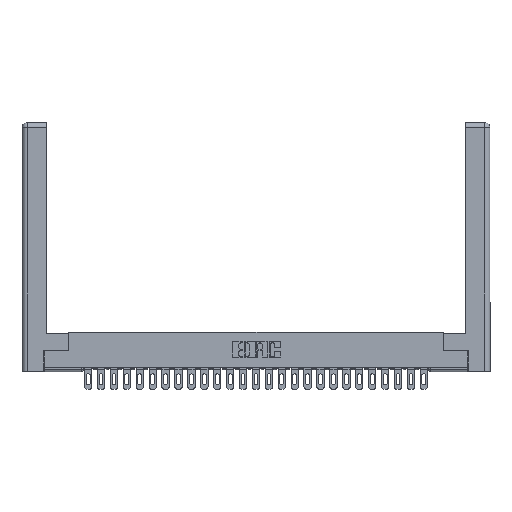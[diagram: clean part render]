
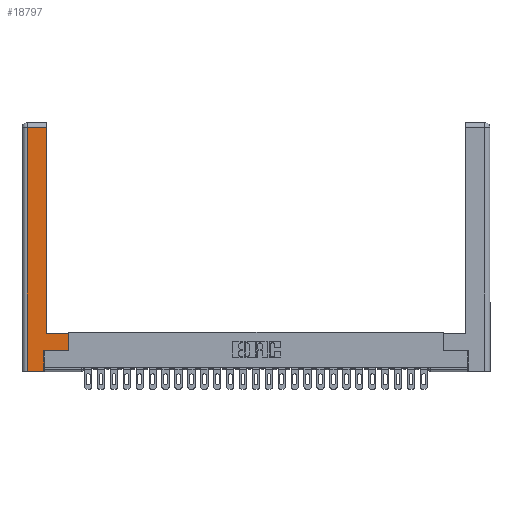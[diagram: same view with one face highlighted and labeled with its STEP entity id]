
A CAD part, top view. The second image highlights one B-rep face of the part: STEP entity #18797.
In plain terms, the highlighted planar face has unit normal (0, 0, 1).
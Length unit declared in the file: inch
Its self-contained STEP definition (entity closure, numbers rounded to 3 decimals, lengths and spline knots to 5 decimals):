
#316 = ORIENTED_EDGE ( 'NONE', *, *, #25225, .T. ) ;
#901 = VECTOR ( 'NONE', #3980, 39.37008 ) ;
#1416 = VERTEX_POINT ( 'NONE', #12453 ) ;
#1665 = VECTOR ( 'NONE', #17833, 39.37008 ) ;
#2496 = VECTOR ( 'NONE', #4115, 39.37008 ) ;
#3275 = VERTEX_POINT ( 'NONE', #26505 ) ;
#3876 = VECTOR ( 'NONE', #23729, 39.37008 ) ;
#3980 = DIRECTION ( 'NONE',  ( 1., 0., 0. ) ) ;
#4115 = DIRECTION ( 'NONE',  ( 0., 1., 0. ) ) ;
#4447 = CARTESIAN_POINT ( 'NONE',  ( 0., 0., 0. ) ) ;
#4611 = ORIENTED_EDGE ( 'NONE', *, *, #17147, .T. ) ;
#5420 = ORIENTED_EDGE ( 'NONE', *, *, #26320, .T. ) ;
#5506 = DIRECTION ( 'NONE',  ( -1., 0., 0. ) ) ;
#5956 = LINE ( 'NONE', #10548, #8752 ) ;
#5998 = LINE ( 'NONE', #8160, #2496 ) ;
#6754 = CARTESIAN_POINT ( 'NONE',  ( 0.565, 0.245, 0. ) ) ;
#7474 = EDGE_CURVE ( 'NONE', #3275, #1416, #10131, .T. ) ;
#7957 = LINE ( 'NONE', #8093, #10818 ) ;
#8093 = CARTESIAN_POINT ( 'NONE',  ( 0.0615, 2.94, 0. ) ) ;
#8160 = CARTESIAN_POINT ( 'NONE',  ( 0.265, 0.245, 0. ) ) ;
#8752 = VECTOR ( 'NONE', #21217, 39.37008 ) ;
#8849 = VECTOR ( 'NONE', #27537, 39.37008 ) ;
#8928 = LINE ( 'NONE', #13110, #1665 ) ;
#9095 = VERTEX_POINT ( 'NONE', #24848 ) ;
#10076 = CARTESIAN_POINT ( 'NONE',  ( 0.295, 3., 0. ) ) ;
#10131 = LINE ( 'NONE', #16468, #8849 ) ;
#10548 = CARTESIAN_POINT ( 'NONE',  ( 0.295, 0.45, 0. ) ) ;
#10818 = VECTOR ( 'NONE', #5506, 39.37008 ) ;
#11807 = LINE ( 'NONE', #10076, #24186 ) ;
#11818 = VERTEX_POINT ( 'NONE', #6754 ) ;
#12041 = EDGE_CURVE ( 'NONE', #11818, #26332, #18823, .T. ) ;
#12094 = ORIENTED_EDGE ( 'NONE', *, *, #12041, .T. ) ;
#12331 = CARTESIAN_POINT ( 'NONE',  ( 0.565, 0.245, 0. ) ) ;
#12453 = CARTESIAN_POINT ( 'NONE',  ( 0.265, 0., 0. ) ) ;
#13110 = CARTESIAN_POINT ( 'NONE',  ( 0.0615, 0., 0. ) ) ;
#13320 = EDGE_CURVE ( 'NONE', #24469, #3275, #8928, .T. ) ;
#13632 = ORIENTED_EDGE ( 'NONE', *, *, #7474, .T. ) ;
#13957 = ORIENTED_EDGE ( 'NONE', *, *, #16183, .T. ) ;
#14445 = CARTESIAN_POINT ( 'NONE',  ( 0.565, 0.45, 0. ) ) ;
#15321 = EDGE_CURVE ( 'NONE', #1416, #18323, #5998, .T. ) ;
#16183 = EDGE_CURVE ( 'NONE', #9095, #24469, #7957, .T. ) ;
#16468 = CARTESIAN_POINT ( 'NONE',  ( 0.265, 0., 0. ) ) ;
#17147 = EDGE_CURVE ( 'NONE', #26369, #9095, #11807, .T. ) ;
#17325 = CARTESIAN_POINT ( 'NONE',  ( 0.265, 0.245, 0. ) ) ;
#17833 = DIRECTION ( 'NONE',  ( 0., -1., 0. ) ) ;
#18323 = VERTEX_POINT ( 'NONE', #17325 ) ;
#18458 = AXIS2_PLACEMENT_3D ( 'NONE', #4447, #22152, #22444 ) ;
#18797 = ADVANCED_FACE ( 'NONE', ( #19981 ), #24311, .F. ) ;
#18823 = LINE ( 'NONE', #25470, #3876 ) ;
#19981 = FACE_OUTER_BOUND ( 'NONE', #28133, .T. ) ;
#21217 = DIRECTION ( 'NONE',  ( -1., 0., 0. ) ) ;
#21897 = ORIENTED_EDGE ( 'NONE', *, *, #13320, .T. ) ;
#22152 = DIRECTION ( 'NONE',  ( 0., 0., -1. ) ) ;
#22444 = DIRECTION ( 'NONE',  ( -1., 0., 0. ) ) ;
#22626 = ORIENTED_EDGE ( 'NONE', *, *, #15321, .T. ) ;
#23729 = DIRECTION ( 'NONE',  ( 0., 1., 0. ) ) ;
#24186 = VECTOR ( 'NONE', #27076, 39.37008 ) ;
#24311 = PLANE ( 'NONE',  #18458 ) ;
#24469 = VERTEX_POINT ( 'NONE', #26247 ) ;
#24848 = CARTESIAN_POINT ( 'NONE',  ( 0.295, 2.94, 0. ) ) ;
#25225 = EDGE_CURVE ( 'NONE', #18323, #11818, #27720, .T. ) ;
#25470 = CARTESIAN_POINT ( 'NONE',  ( 0.565, 0.45, 0. ) ) ;
#26247 = CARTESIAN_POINT ( 'NONE',  ( 0.0615, 2.94, 0. ) ) ;
#26320 = EDGE_CURVE ( 'NONE', #26332, #26369, #5956, .T. ) ;
#26332 = VERTEX_POINT ( 'NONE', #14445 ) ;
#26369 = VERTEX_POINT ( 'NONE', #28109 ) ;
#26505 = CARTESIAN_POINT ( 'NONE',  ( 0.0615, 0., 0. ) ) ;
#27076 = DIRECTION ( 'NONE',  ( 0., 1., 0. ) ) ;
#27537 = DIRECTION ( 'NONE',  ( 1., 0., 0. ) ) ;
#27720 = LINE ( 'NONE', #12331, #901 ) ;
#28109 = CARTESIAN_POINT ( 'NONE',  ( 0.295, 0.45, 0. ) ) ;
#28133 = EDGE_LOOP ( 'NONE', ( #4611, #13957, #21897, #13632, #22626, #316, #12094, #5420 ) ) ;
